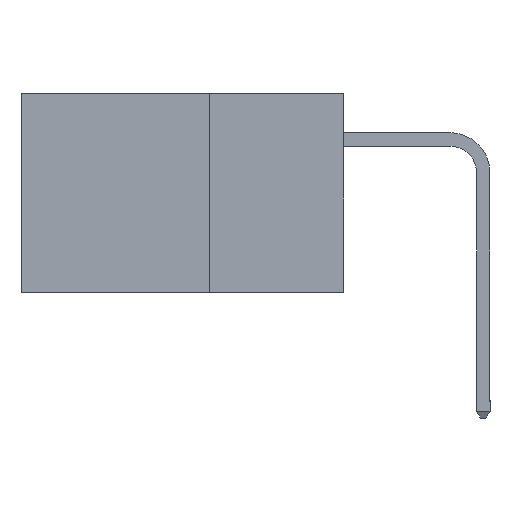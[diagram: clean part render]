
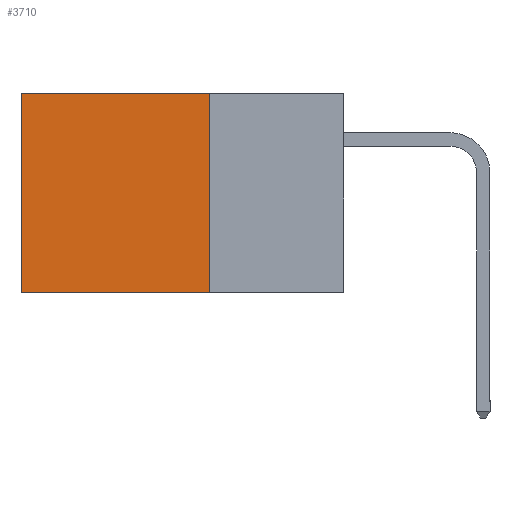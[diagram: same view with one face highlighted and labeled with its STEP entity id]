
A CAD part, left-side view. The second image highlights one B-rep face of the part: STEP entity #3710.
In plain terms, the highlighted planar face has unit normal (-1, 0, 0).
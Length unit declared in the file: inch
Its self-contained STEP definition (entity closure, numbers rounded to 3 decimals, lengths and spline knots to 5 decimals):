
#27 = ORIENTED_EDGE ( 'NONE', *, *, #2488, .T. ) ;
#1322 = CARTESIAN_POINT ( 'NONE',  ( 0.2615, 0.6, 0. ) ) ;
#1397 = LINE ( 'NONE', #3586, #9174 ) ;
#1561 = VERTEX_POINT ( 'NONE', #1322 ) ;
#1573 = LINE ( 'NONE', #8146, #5932 ) ;
#1694 = VECTOR ( 'NONE', #5415, 39.37008 ) ;
#1752 = DIRECTION ( 'NONE',  ( 0., 1., 0. ) ) ;
#2488 = EDGE_CURVE ( 'NONE', #1561, #9074, #1573, .T. ) ;
#2507 = EDGE_CURVE ( 'NONE', #9427, #1561, #9802, .T. ) ;
#3586 = CARTESIAN_POINT ( 'NONE',  ( 0.2615, 0.25, -0.37 ) ) ;
#3710 = ADVANCED_FACE ( 'NONE', ( #9322 ), #4398, .F. ) ;
#3902 = EDGE_CURVE ( 'NONE', #9427, #8656, #9915, .T. ) ;
#4224 = AXIS2_PLACEMENT_3D ( 'NONE', #6760, #9863, #5205 ) ;
#4301 = ORIENTED_EDGE ( 'NONE', *, *, #4818, .F. ) ;
#4398 = PLANE ( 'NONE',  #4224 ) ;
#4818 = EDGE_CURVE ( 'NONE', #8656, #9074, #1397, .T. ) ;
#5025 = CARTESIAN_POINT ( 'NONE',  ( 0.2615, 0.25, 0. ) ) ;
#5188 = DIRECTION ( 'NONE',  ( 0., 1., 0. ) ) ;
#5205 = DIRECTION ( 'NONE',  ( 0., 0., -1. ) ) ;
#5415 = DIRECTION ( 'NONE',  ( 0., 0., -1. ) ) ;
#5490 = CARTESIAN_POINT ( 'NONE',  ( 0.2615, 0.25, 0. ) ) ;
#5595 = ORIENTED_EDGE ( 'NONE', *, *, #3902, .F. ) ;
#5932 = VECTOR ( 'NONE', #8916, 39.37008 ) ;
#5972 = ORIENTED_EDGE ( 'NONE', *, *, #2507, .T. ) ;
#6218 = CARTESIAN_POINT ( 'NONE',  ( 0.2615, 0.25, -0.37 ) ) ;
#6760 = CARTESIAN_POINT ( 'NONE',  ( 0.2615, 0.25, -0.37 ) ) ;
#7995 = VECTOR ( 'NONE', #1752, 39.37008 ) ;
#8146 = CARTESIAN_POINT ( 'NONE',  ( 0.2615, 0.6, -0.37 ) ) ;
#8656 = VERTEX_POINT ( 'NONE', #9390 ) ;
#8767 = EDGE_LOOP ( 'NONE', ( #27, #4301, #5595, #5972 ) ) ;
#8916 = DIRECTION ( 'NONE',  ( 0., 0., -1. ) ) ;
#8956 = CARTESIAN_POINT ( 'NONE',  ( 0.2615, 0.6, -0.37 ) ) ;
#9074 = VERTEX_POINT ( 'NONE', #8956 ) ;
#9174 = VECTOR ( 'NONE', #5188, 39.37008 ) ;
#9322 = FACE_OUTER_BOUND ( 'NONE', #8767, .T. ) ;
#9390 = CARTESIAN_POINT ( 'NONE',  ( 0.2615, 0.25, -0.37 ) ) ;
#9427 = VERTEX_POINT ( 'NONE', #5490 ) ;
#9802 = LINE ( 'NONE', #5025, #7995 ) ;
#9863 = DIRECTION ( 'NONE',  ( 1., 0., 0. ) ) ;
#9915 = LINE ( 'NONE', #6218, #1694 ) ;
